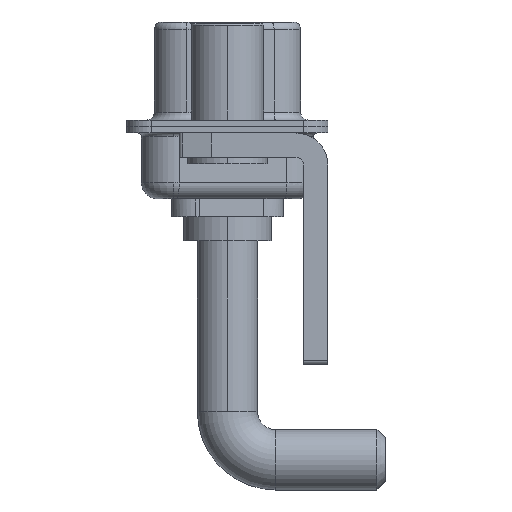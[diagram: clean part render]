
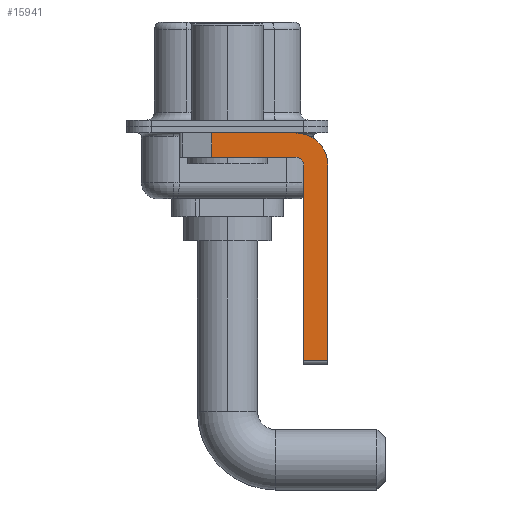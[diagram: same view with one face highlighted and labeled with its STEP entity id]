
A CAD part, left-side view. The second image highlights one B-rep face of the part: STEP entity #15941.
In plain terms, the highlighted planar face has unit normal (-1, 0, 0).
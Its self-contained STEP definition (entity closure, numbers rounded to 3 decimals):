
#281 = ORIENTED_EDGE ( 'NONE', *, *, #9342, .F. ) ;
#542 = VECTOR ( 'NONE', #17205, 1000. ) ;
#772 = ORIENTED_EDGE ( 'NONE', *, *, #4829, .T. ) ;
#878 = PLANE ( 'NONE',  #4167 ) ;
#1095 = VERTEX_POINT ( 'NONE', #14335 ) ;
#1368 = CARTESIAN_POINT ( 'NONE',  ( -2.9, -4.25, -1.9 ) ) ;
#1381 = LINE ( 'NONE', #12598, #542 ) ;
#1425 = EDGE_CURVE ( 'NONE', #1095, #3279, #3658, .T. ) ;
#1495 = CARTESIAN_POINT ( 'NONE',  ( -2.9, -4.75, -14.55 ) ) ;
#1784 = LINE ( 'NONE', #14509, #10315 ) ;
#3273 = DIRECTION ( 'NONE',  ( 0., 0., 1. ) ) ;
#3279 = VERTEX_POINT ( 'NONE', #13972 ) ;
#3325 = VERTEX_POINT ( 'NONE', #12376 ) ;
#3578 = CARTESIAN_POINT ( 'NONE',  ( -2.9, -4.25, -1.9 ) ) ;
#3658 = LINE ( 'NONE', #9410, #6576 ) ;
#4136 = ORIENTED_EDGE ( 'NONE', *, *, #14269, .T. ) ;
#4155 = VECTOR ( 'NONE', #11252, 1000. ) ;
#4167 = AXIS2_PLACEMENT_3D ( 'NONE', #15091, #9522, #12370 ) ;
#4650 = DIRECTION ( 'NONE',  ( 0., 0., -1. ) ) ;
#4829 = EDGE_CURVE ( 'NONE', #13711, #9736, #17266, .T. ) ;
#4869 = AXIS2_PLACEMENT_3D ( 'NONE', #11823, #7567, #4650 ) ;
#5234 = DIRECTION ( 'NONE',  ( 0., 0., 1. ) ) ;
#5873 = CARTESIAN_POINT ( 'NONE',  ( -2.9, 0.978, -1.9 ) ) ;
#6559 = CARTESIAN_POINT ( 'NONE',  ( -2.9, -4.25, -2.4 ) ) ;
#6576 = VECTOR ( 'NONE', #15161, 1000. ) ;
#6702 = EDGE_CURVE ( 'NONE', #14948, #1095, #16016, .T. ) ;
#7451 = ORIENTED_EDGE ( 'NONE', *, *, #7865, .F. ) ;
#7567 = DIRECTION ( 'NONE',  ( 1., 0., 0. ) ) ;
#7865 = EDGE_CURVE ( 'NONE', #3325, #10042, #13920, .T. ) ;
#9329 = DIRECTION ( 'NONE',  ( 0., 1., 0. ) ) ;
#9338 = FACE_OUTER_BOUND ( 'NONE', #18327, .T. ) ;
#9342 = EDGE_CURVE ( 'NONE', #13318, #3325, #1784, .T. ) ;
#9410 = CARTESIAN_POINT ( 'NONE',  ( -2.9, -6.25, -2.4 ) ) ;
#9522 = DIRECTION ( 'NONE',  ( 1., 0., 0. ) ) ;
#9736 = VERTEX_POINT ( 'NONE', #14386 ) ;
#10042 = VERTEX_POINT ( 'NONE', #1368 ) ;
#10091 = ORIENTED_EDGE ( 'NONE', *, *, #6702, .F. ) ;
#10315 = VECTOR ( 'NONE', #3273, 1000. ) ;
#10719 = CARTESIAN_POINT ( 'NONE',  ( -2.9, -4.25, -0.4 ) ) ;
#11252 = DIRECTION ( 'NONE',  ( 0., -1., 0. ) ) ;
#11823 = CARTESIAN_POINT ( 'NONE',  ( -2.9, -4.25, -2.4 ) ) ;
#12060 = EDGE_CURVE ( 'NONE', #10042, #9736, #16598, .T. ) ;
#12370 = DIRECTION ( 'NONE',  ( 0., 0., -1. ) ) ;
#12376 = CARTESIAN_POINT ( 'NONE',  ( -2.9, -4.75, -2.4 ) ) ;
#12393 = DIRECTION ( 'NONE',  ( -1., 0., 0. ) ) ;
#12493 = VECTOR ( 'NONE', #9329, 1000. ) ;
#12598 = CARTESIAN_POINT ( 'NONE',  ( -2.9, 3., -0.4 ) ) ;
#13318 = VERTEX_POINT ( 'NONE', #1495 ) ;
#13711 = VERTEX_POINT ( 'NONE', #16922 ) ;
#13920 = CIRCLE ( 'NONE', #18117, 0.5 ) ;
#13972 = CARTESIAN_POINT ( 'NONE',  ( -2.9, -6.25, -14.55 ) ) ;
#14169 = LINE ( 'NONE', #18398, #4155 ) ;
#14269 = EDGE_CURVE ( 'NONE', #13318, #3279, #14169, .T. ) ;
#14335 = CARTESIAN_POINT ( 'NONE',  ( -2.9, -6.25, -2.4 ) ) ;
#14386 = CARTESIAN_POINT ( 'NONE',  ( -2.9, 0.978, -1.9 ) ) ;
#14509 = CARTESIAN_POINT ( 'NONE',  ( -2.9, -4.75, -14.8 ) ) ;
#14863 = ORIENTED_EDGE ( 'NONE', *, *, #12060, .F. ) ;
#14948 = VERTEX_POINT ( 'NONE', #10719 ) ;
#15091 = CARTESIAN_POINT ( 'NONE',  ( -2.9, -4.25, -2.4 ) ) ;
#15161 = DIRECTION ( 'NONE',  ( 0., 0., -1. ) ) ;
#15194 = EDGE_CURVE ( 'NONE', #13711, #14948, #1381, .T. ) ;
#15281 = ORIENTED_EDGE ( 'NONE', *, *, #15194, .F. ) ;
#15766 = DIRECTION ( 'NONE',  ( 0., 0., -1. ) ) ;
#15941 = ADVANCED_FACE ( 'NONE', ( #9338 ), #878, .F. ) ;
#15950 = VECTOR ( 'NONE', #15766, 1000. ) ;
#16016 = CIRCLE ( 'NONE', #4869, 2. ) ;
#16598 = LINE ( 'NONE', #3578, #12493 ) ;
#16922 = CARTESIAN_POINT ( 'NONE',  ( -2.9, 0.978, -0.4 ) ) ;
#17205 = DIRECTION ( 'NONE',  ( 0., -1., 0. ) ) ;
#17266 = LINE ( 'NONE', #5873, #15950 ) ;
#18117 = AXIS2_PLACEMENT_3D ( 'NONE', #6559, #12393, #5234 ) ;
#18143 = ORIENTED_EDGE ( 'NONE', *, *, #1425, .F. ) ;
#18327 = EDGE_LOOP ( 'NONE', ( #15281, #772, #14863, #7451, #281, #4136, #18143, #10091 ) ) ;
#18398 = CARTESIAN_POINT ( 'NONE',  ( -2.9, -4.25, -14.55 ) ) ;
